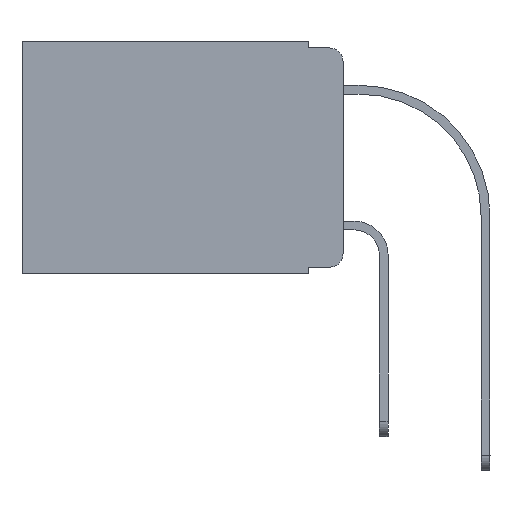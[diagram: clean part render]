
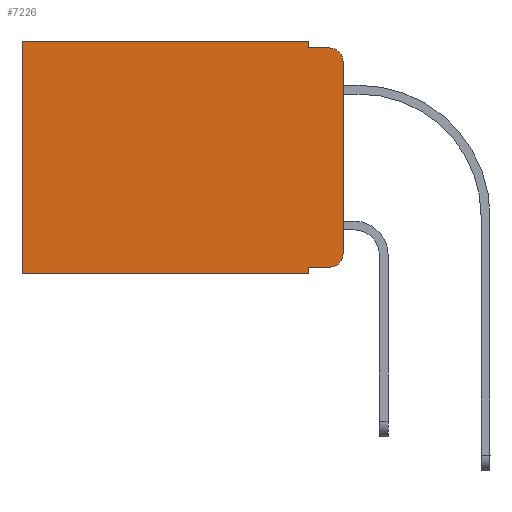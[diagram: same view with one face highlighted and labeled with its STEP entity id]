
A CAD part, left-side view. The second image highlights one B-rep face of the part: STEP entity #7226.
In plain terms, the highlighted planar face has unit normal (-1, 0, 0).
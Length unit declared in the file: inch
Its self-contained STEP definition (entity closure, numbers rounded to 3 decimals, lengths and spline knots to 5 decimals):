
#126 = LINE ( 'NONE', #6899, #12778 ) ;
#260 = DIRECTION ( 'NONE',  ( 0., -1., 0. ) ) ;
#857 = LINE ( 'NONE', #11874, #11138 ) ;
#1046 = EDGE_CURVE ( 'NONE', #16359, #8695, #5410, .T. ) ;
#1179 = EDGE_CURVE ( 'NONE', #5782, #1748, #3392, .T. ) ;
#1317 = VECTOR ( 'NONE', #11961, 39.37008 ) ;
#1583 = EDGE_CURVE ( 'NONE', #16650, #4168, #16004, .T. ) ;
#1748 = VERTEX_POINT ( 'NONE', #11181 ) ;
#1820 = DIRECTION ( 'NONE',  ( 1., 0., 0. ) ) ;
#1911 = VECTOR ( 'NONE', #6564, 39.37008 ) ;
#1987 = CARTESIAN_POINT ( 'NONE',  ( 0.298, 0.473, 0. ) ) ;
#2110 = ORIENTED_EDGE ( 'NONE', *, *, #11080, .F. ) ;
#2177 = CARTESIAN_POINT ( 'NONE',  ( 0.298, 0.051, 0. ) ) ;
#2190 = CARTESIAN_POINT ( 'NONE',  ( 0.298, 0.051, -0.01 ) ) ;
#2938 = ORIENTED_EDGE ( 'NONE', *, *, #14132, .T. ) ;
#2974 = DIRECTION ( 'NONE',  ( -1., 0., 0. ) ) ;
#3073 = CARTESIAN_POINT ( 'NONE',  ( 0.298, 0.02, -0.313 ) ) ;
#3303 = AXIS2_PLACEMENT_3D ( 'NONE', #9550, #12434, #5567 ) ;
#3392 = CIRCLE ( 'NONE', #13489, 0.02 ) ;
#3681 = VECTOR ( 'NONE', #14184, 39.37008 ) ;
#3730 = DIRECTION ( 'NONE',  ( 0., 1., 0. ) ) ;
#4068 = EDGE_CURVE ( 'NONE', #14033, #15046, #126, .T. ) ;
#4168 = VERTEX_POINT ( 'NONE', #12939 ) ;
#5110 = ORIENTED_EDGE ( 'NONE', *, *, #5874, .T. ) ;
#5214 = VECTOR ( 'NONE', #260, 39.37008 ) ;
#5410 = LINE ( 'NONE', #6760, #12046 ) ;
#5567 = DIRECTION ( 'NONE',  ( 0., 0., -1. ) ) ;
#5766 = CARTESIAN_POINT ( 'NONE',  ( 0.298, 0.051, -0.01 ) ) ;
#5782 = VERTEX_POINT ( 'NONE', #5882 ) ;
#5828 = CARTESIAN_POINT ( 'NONE',  ( 0.298, 0.051, -0.333 ) ) ;
#5874 = EDGE_CURVE ( 'NONE', #9799, #5782, #15556, .T. ) ;
#5882 = CARTESIAN_POINT ( 'NONE',  ( 0.298, 0.02, -0.333 ) ) ;
#5995 = ORIENTED_EDGE ( 'NONE', *, *, #1046, .F. ) ;
#5999 = EDGE_CURVE ( 'NONE', #9799, #14033, #7953, .T. ) ;
#6515 = ORIENTED_EDGE ( 'NONE', *, *, #4068, .F. ) ;
#6564 = DIRECTION ( 'NONE',  ( 0., 0., -1. ) ) ;
#6760 = CARTESIAN_POINT ( 'NONE',  ( 0.298, 0.051, 0. ) ) ;
#6899 = CARTESIAN_POINT ( 'NONE',  ( 0.298, 0., -0.343 ) ) ;
#7226 = ADVANCED_FACE ( 'NONE', ( #10056 ), #16741, .F. ) ;
#7625 = LINE ( 'NONE', #12047, #1317 ) ;
#7953 = LINE ( 'NONE', #2177, #12917 ) ;
#8013 = CARTESIAN_POINT ( 'NONE',  ( 0.298, 0., 0. ) ) ;
#8162 = DIRECTION ( 'NONE',  ( 0., 1., 0. ) ) ;
#8254 = EDGE_LOOP ( 'NONE', ( #2110, #11784, #10037, #5995, #2938, #10831, #6515, #12509, #5110, #8349 ) ) ;
#8349 = ORIENTED_EDGE ( 'NONE', *, *, #1179, .T. ) ;
#8683 = CARTESIAN_POINT ( 'NONE',  ( 0.298, 0.051, -0.333 ) ) ;
#8695 = VERTEX_POINT ( 'NONE', #2190 ) ;
#8894 = CARTESIAN_POINT ( 'NONE',  ( 0.298, 0.051, -0.343 ) ) ;
#9365 = LINE ( 'NONE', #8013, #1911 ) ;
#9399 = EDGE_CURVE ( 'NONE', #8695, #4168, #10018, .T. ) ;
#9550 = CARTESIAN_POINT ( 'NONE',  ( 0.298, 0.02, -0.03 ) ) ;
#9799 = VERTEX_POINT ( 'NONE', #5828 ) ;
#10018 = LINE ( 'NONE', #5766, #5214 ) ;
#10037 = ORIENTED_EDGE ( 'NONE', *, *, #9399, .F. ) ;
#10056 = FACE_OUTER_BOUND ( 'NONE', #8254, .T. ) ;
#10831 = ORIENTED_EDGE ( 'NONE', *, *, #14060, .T. ) ;
#11080 = EDGE_CURVE ( 'NONE', #16650, #1748, #9365, .T. ) ;
#11138 = VECTOR ( 'NONE', #3730, 39.37008 ) ;
#11181 = CARTESIAN_POINT ( 'NONE',  ( 0.298, 0., -0.313 ) ) ;
#11784 = ORIENTED_EDGE ( 'NONE', *, *, #1583, .T. ) ;
#11860 = CARTESIAN_POINT ( 'NONE',  ( 0.298, 0.051, 0. ) ) ;
#11874 = CARTESIAN_POINT ( 'NONE',  ( 0.298, 0., 0. ) ) ;
#11961 = DIRECTION ( 'NONE',  ( 0., 0., -1. ) ) ;
#12046 = VECTOR ( 'NONE', #12365, 39.37008 ) ;
#12047 = CARTESIAN_POINT ( 'NONE',  ( 0.298, 0.473, 0. ) ) ;
#12365 = DIRECTION ( 'NONE',  ( 0., 0., -1. ) ) ;
#12434 = DIRECTION ( 'NONE',  ( -1., 0., 0. ) ) ;
#12509 = ORIENTED_EDGE ( 'NONE', *, *, #5999, .F. ) ;
#12778 = VECTOR ( 'NONE', #8162, 39.37008 ) ;
#12917 = VECTOR ( 'NONE', #13460, 39.37008 ) ;
#12939 = CARTESIAN_POINT ( 'NONE',  ( 0.298, 0.02, -0.01 ) ) ;
#13460 = DIRECTION ( 'NONE',  ( 0., 0., -1. ) ) ;
#13489 = AXIS2_PLACEMENT_3D ( 'NONE', #3073, #2974, #16711 ) ;
#14033 = VERTEX_POINT ( 'NONE', #8894 ) ;
#14060 = EDGE_CURVE ( 'NONE', #14397, #15046, #7625, .T. ) ;
#14132 = EDGE_CURVE ( 'NONE', #16359, #14397, #857, .T. ) ;
#14184 = DIRECTION ( 'NONE',  ( 0., -1., 0. ) ) ;
#14397 = VERTEX_POINT ( 'NONE', #1987 ) ;
#15046 = VERTEX_POINT ( 'NONE', #15148 ) ;
#15148 = CARTESIAN_POINT ( 'NONE',  ( 0.298, 0.473, -0.343 ) ) ;
#15556 = LINE ( 'NONE', #8683, #3681 ) ;
#15562 = CARTESIAN_POINT ( 'NONE',  ( 0.298, 0., 0. ) ) ;
#16004 = CIRCLE ( 'NONE', #3303, 0.02 ) ;
#16359 = VERTEX_POINT ( 'NONE', #11860 ) ;
#16547 = CARTESIAN_POINT ( 'NONE',  ( 0.298, 0., -0.03 ) ) ;
#16650 = VERTEX_POINT ( 'NONE', #16547 ) ;
#16711 = DIRECTION ( 'NONE',  ( 0., 0., -1. ) ) ;
#16741 = PLANE ( 'NONE',  #17150 ) ;
#16831 = DIRECTION ( 'NONE',  ( 0., 0., -1. ) ) ;
#17150 = AXIS2_PLACEMENT_3D ( 'NONE', #15562, #1820, #16831 ) ;
